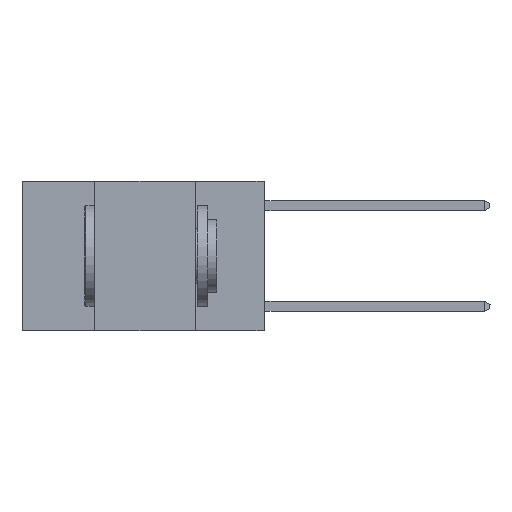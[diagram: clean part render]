
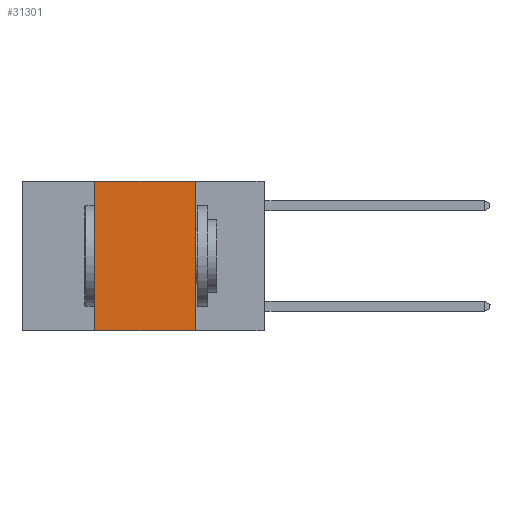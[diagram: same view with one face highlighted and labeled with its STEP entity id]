
A CAD part, left-side view. The second image highlights one B-rep face of the part: STEP entity #31301.
In plain terms, the highlighted planar face has unit normal (-1, 0, 0).
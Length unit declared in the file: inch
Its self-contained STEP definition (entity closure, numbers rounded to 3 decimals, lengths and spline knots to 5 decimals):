
#2236 = CARTESIAN_POINT ( 'NONE',  ( 0., 0.6, 0. ) ) ;
#3540 = ORIENTED_EDGE ( 'NONE', *, *, #17360, .T. ) ;
#5600 = ORIENTED_EDGE ( 'NONE', *, *, #21507, .F. ) ;
#5815 = VERTEX_POINT ( 'NONE', #6852 ) ;
#6430 = VECTOR ( 'NONE', #28211, 39.37008 ) ;
#6852 = CARTESIAN_POINT ( 'NONE',  ( 0., 0.17, 0. ) ) ;
#7100 = VECTOR ( 'NONE', #28971, 39.37008 ) ;
#7207 = CARTESIAN_POINT ( 'NONE',  ( 0., 0.42, -0.37 ) ) ;
#8894 = EDGE_CURVE ( 'NONE', #5815, #28195, #24157, .T. ) ;
#9213 = DIRECTION ( 'NONE',  ( 1., 0., 0. ) ) ;
#9353 = CARTESIAN_POINT ( 'NONE',  ( 0., 0.6, 0. ) ) ;
#9883 = DIRECTION ( 'NONE',  ( 0., 0., -1. ) ) ;
#10080 = LINE ( 'NONE', #15589, #6430 ) ;
#10605 = CARTESIAN_POINT ( 'NONE',  ( 0., 0.6, -0.37 ) ) ;
#10992 = CARTESIAN_POINT ( 'NONE',  ( 0., 0.42, 0. ) ) ;
#12200 = FACE_OUTER_BOUND ( 'NONE', #13361, .T. ) ;
#13361 = EDGE_LOOP ( 'NONE', ( #13995, #5600, #13603, #3540 ) ) ;
#13603 = ORIENTED_EDGE ( 'NONE', *, *, #30996, .F. ) ;
#13995 = ORIENTED_EDGE ( 'NONE', *, *, #8894, .F. ) ;
#14541 = VERTEX_POINT ( 'NONE', #7207 ) ;
#15589 = CARTESIAN_POINT ( 'NONE',  ( 0., 0.42, 0. ) ) ;
#17360 = EDGE_CURVE ( 'NONE', #14541, #28195, #20425, .T. ) ;
#19355 = LINE ( 'NONE', #9353, #24462 ) ;
#20425 = LINE ( 'NONE', #10605, #29163 ) ;
#20563 = VERTEX_POINT ( 'NONE', #10992 ) ;
#21507 = EDGE_CURVE ( 'NONE', #20563, #5815, #19355, .T. ) ;
#21891 = AXIS2_PLACEMENT_3D ( 'NONE', #2236, #9213, #9883 ) ;
#22853 = CARTESIAN_POINT ( 'NONE',  ( 0., 0.17, -0.37 ) ) ;
#24157 = LINE ( 'NONE', #31773, #7100 ) ;
#24462 = VECTOR ( 'NONE', #24517, 39.37008 ) ;
#24517 = DIRECTION ( 'NONE',  ( 0., -1., 0. ) ) ;
#28195 = VERTEX_POINT ( 'NONE', #22853 ) ;
#28211 = DIRECTION ( 'NONE',  ( 0., 0., 1. ) ) ;
#28971 = DIRECTION ( 'NONE',  ( 0., 0., -1. ) ) ;
#29163 = VECTOR ( 'NONE', #30535, 39.37008 ) ;
#30535 = DIRECTION ( 'NONE',  ( 0., -1., 0. ) ) ;
#30996 = EDGE_CURVE ( 'NONE', #14541, #20563, #10080, .T. ) ;
#31301 = ADVANCED_FACE ( 'NONE', ( #12200 ), #32004, .F. ) ;
#31773 = CARTESIAN_POINT ( 'NONE',  ( 0., 0.17, 0. ) ) ;
#32004 = PLANE ( 'NONE',  #21891 ) ;
